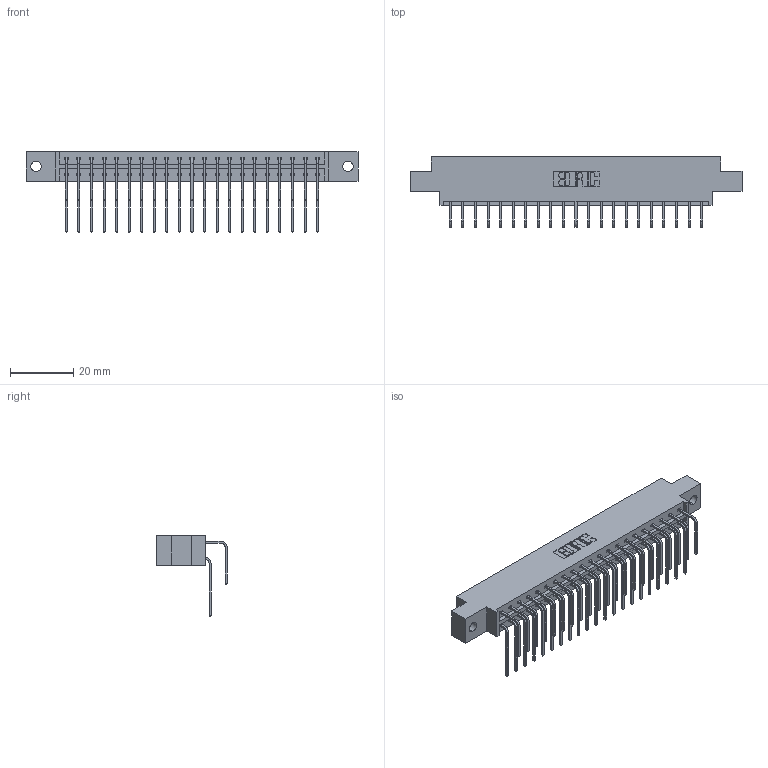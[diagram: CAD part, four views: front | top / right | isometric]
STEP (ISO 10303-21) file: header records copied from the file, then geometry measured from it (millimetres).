
FILE_DESCRIPTION (( 'STEP AP203' ), '1' );
FILE_NAME ('833-042-558-802.STEP', '2020-06-03T22:37:21', ( '' ), ( '' ), 'SwSTEP 2.0', 'SolidWorks 2020', '' );
FILE_SCHEMA (( 'CONFIG_CONTROL_DESIGN' ));
Length unit declared in the file: inch
Products named in the file (4): 345-292-001_558 559 Tail - 1; 833-042-558-802; 833 Part_Offset - .128 Dia; 345-292-001_558 Tail - 2
Assembly tree (43 placements, depth 2):
  833-042-558-802
    833 Part_Offset - .128 Dia
    345-292-001_558 559 Tail - 1  x21
    345-292-001_558 Tail - 2  x21
Bounding box: 104.75 x 22.17 x 25.53 mm (x, y, z)
Volume: 10475.8 mm3; surface area: 13313.6 mm2
Topology: 43 solids, 43 shells, 2386 faces, 7085 edges, 4666 vertices
Faces by surface type: plane 1670, cylinder 716
Entity records: 18145 total; most frequent: CARTESIAN_POINT 3085, ORIENTED_EDGE 2970, DIRECTION 2653, EDGE_CURVE 1485, LINE 1317, VECTOR 1317, VERTEX_POINT 986, AXIS2_PLACEMENT_3D 668
